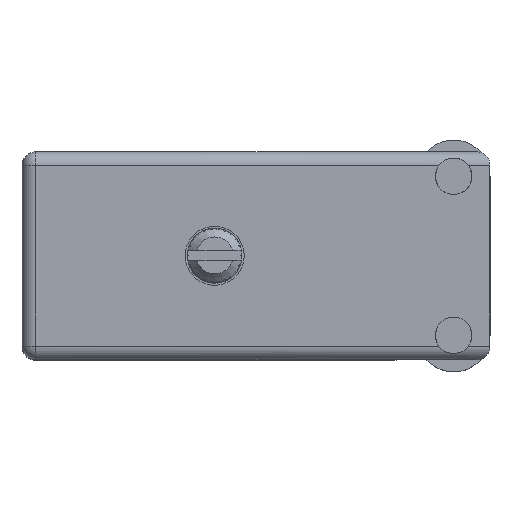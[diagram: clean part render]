
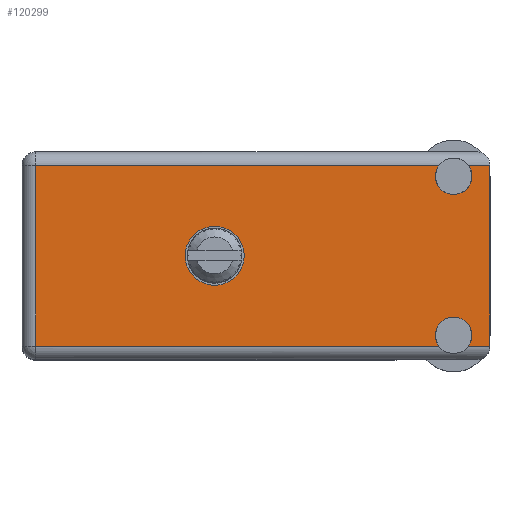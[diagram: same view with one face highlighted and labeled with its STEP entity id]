
A CAD part, top view. The second image highlights one B-rep face of the part: STEP entity #120299.
In plain terms, the highlighted face is planar.
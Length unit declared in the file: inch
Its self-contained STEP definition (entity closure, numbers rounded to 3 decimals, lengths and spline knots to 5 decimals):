
#90 = EDGE_CURVE ( 'NONE', #178435, #7572, #18110, .T. ) ;
#620 = AXIS2_PLACEMENT_3D ( 'NONE', #87096, #186670, #1561 ) ;
#1392 = DIRECTION ( 'NONE',  ( -1., 0., 0. ) ) ;
#1561 = DIRECTION ( 'NONE',  ( 0., 0., 1. ) ) ;
#3412 = FACE_OUTER_BOUND ( 'NONE', #26400, .T. ) ;
#4773 = LINE ( 'NONE', #108244, #90241 ) ;
#5394 = DIRECTION ( 'NONE',  ( 0., 0., 1. ) ) ;
#7572 = VERTEX_POINT ( 'NONE', #61133 ) ;
#8614 = CARTESIAN_POINT ( 'NONE',  ( 0.047, 0.906, -0.668 ) ) ;
#11567 = EDGE_CURVE ( 'NONE', #169026, #52954, #19464, .T. ) ;
#12665 = CARTESIAN_POINT ( 'NONE',  ( 1.609, 0.906, -0.668 ) ) ;
#14396 = VERTEX_POINT ( 'NONE', #134176 ) ;
#15865 = DIRECTION ( 'NONE',  ( 0., 0., 1. ) ) ;
#18110 = LINE ( 'NONE', #146766, #166733 ) ;
#18716 = ORIENTED_EDGE ( 'NONE', *, *, #126770, .F. ) ;
#19232 = CARTESIAN_POINT ( 'NONE',  ( 0.047, 0.906, -0.715 ) ) ;
#19464 = LINE ( 'NONE', #115855, #138938 ) ;
#19802 = CARTESIAN_POINT ( 'NONE',  ( 0.047, 0.906, -0.047 ) ) ;
#20784 = CARTESIAN_POINT ( 'NONE',  ( 0.6625, 0.906, -0.3575 ) ) ;
#24132 = VERTEX_POINT ( 'NONE', #49599 ) ;
#24879 = EDGE_CURVE ( 'NONE', #169026, #179989, #95644, .T. ) ;
#25319 = ORIENTED_EDGE ( 'NONE', *, *, #183548, .T. ) ;
#26400 = EDGE_LOOP ( 'NONE', ( #163845, #70627, #18716, #25319, #99517, #118230, #136854, #134449, #92781, #168842 ) ) ;
#27585 = DIRECTION ( 'NONE',  ( 0., 1., 0. ) ) ;
#30306 = CARTESIAN_POINT ( 'NONE',  ( 1.484, 0.906, -0.631 ) ) ;
#31467 = DIRECTION ( 'NONE',  ( 0., 0., 1. ) ) ;
#36106 = DIRECTION ( 'NONE',  ( 0., 0., 1. ) ) ;
#36639 = DIRECTION ( 'NONE',  ( 1., 0., 0. ) ) ;
#36989 = VECTOR ( 'NONE', #36639, 39.37008 ) ;
#39320 = LINE ( 'NONE', #150470, #36989 ) ;
#39369 = CARTESIAN_POINT ( 'NONE',  ( 0.6625, 0.906, -0.256 ) ) ;
#44323 = CIRCLE ( 'NONE', #620, 0.1015 ) ;
#47089 = ORIENTED_EDGE ( 'NONE', *, *, #61218, .F. ) ;
#48725 = CARTESIAN_POINT ( 'NONE',  ( 1.484, 0.906, -0.084 ) ) ;
#49599 = CARTESIAN_POINT ( 'NONE',  ( 1.43363, 0.906, -0.668 ) ) ;
#52759 = EDGE_CURVE ( 'NONE', #142953, #179690, #44323, .T. ) ;
#52954 = VERTEX_POINT ( 'NONE', #86957 ) ;
#54761 = DIRECTION ( 'NONE',  ( -1., 0., 0. ) ) ;
#55183 = DIRECTION ( 'NONE',  ( 0., 0., 1. ) ) ;
#57534 = VECTOR ( 'NONE', #1392, 39.37008 ) ;
#61133 = CARTESIAN_POINT ( 'NONE',  ( 1.43363, 0.906, -0.047 ) ) ;
#61218 = EDGE_CURVE ( 'NONE', #179690, #142953, #103484, .T. ) ;
#63810 = CARTESIAN_POINT ( 'NONE',  ( 1.53437, 0.906, -0.668 ) ) ;
#69280 = CIRCLE ( 'NONE', #184212, 0.0625 ) ;
#69615 = VECTOR ( 'NONE', #5394, 39.37008 ) ;
#70627 = ORIENTED_EDGE ( 'NONE', *, *, #115244, .F. ) ;
#73059 = AXIS2_PLACEMENT_3D ( 'NONE', #85250, #141267, #55183 ) ;
#77898 = EDGE_CURVE ( 'NONE', #110875, #178435, #107868, .T. ) ;
#82632 = AXIS2_PLACEMENT_3D ( 'NONE', #20784, #120786, #150272 ) ;
#85250 = CARTESIAN_POINT ( 'NONE',  ( 1.484, 0.906, -0.631 ) ) ;
#86957 = CARTESIAN_POINT ( 'NONE',  ( 1.609, 0.906, -0.047 ) ) ;
#87096 = CARTESIAN_POINT ( 'NONE',  ( 0.6625, 0.906, -0.3575 ) ) ;
#87208 = EDGE_CURVE ( 'NONE', #24132, #117075, #146829, .T. ) ;
#90241 = VECTOR ( 'NONE', #54761, 39.37008 ) ;
#92781 = ORIENTED_EDGE ( 'NONE', *, *, #129694, .T. ) ;
#95644 = LINE ( 'NONE', #117705, #57534 ) ;
#99517 = ORIENTED_EDGE ( 'NONE', *, *, #11567, .F. ) ;
#102004 = DIRECTION ( 'NONE',  ( 0., 0., 1. ) ) ;
#103484 = CIRCLE ( 'NONE', #82632, 0.1015 ) ;
#103827 = DIRECTION ( 'NONE',  ( 0., 1., 0. ) ) ;
#105420 = VERTEX_POINT ( 'NONE', #155759 ) ;
#107868 = LINE ( 'NONE', #19232, #69615 ) ;
#108244 = CARTESIAN_POINT ( 'NONE',  ( 0., 0.906, -0.668 ) ) ;
#110875 = VERTEX_POINT ( 'NONE', #8614 ) ;
#114129 = AXIS2_PLACEMENT_3D ( 'NONE', #30306, #130334, #15865 ) ;
#114368 = EDGE_CURVE ( 'NONE', #117075, #179989, #114400, .T. ) ;
#114400 = CIRCLE ( 'NONE', #114129, 0.0625 ) ;
#115244 = EDGE_CURVE ( 'NONE', #105420, #7572, #69280, .T. ) ;
#115615 = CARTESIAN_POINT ( 'NONE',  ( 0., 0.906, -0.715 ) ) ;
#115855 = CARTESIAN_POINT ( 'NONE',  ( 1.609, 0.906, 0. ) ) ;
#117075 = VERTEX_POINT ( 'NONE', #178311 ) ;
#117233 = DIRECTION ( 'NONE',  ( 1., 0., 0. ) ) ;
#117705 = CARTESIAN_POINT ( 'NONE',  ( 0., 0.906, -0.668 ) ) ;
#118230 = ORIENTED_EDGE ( 'NONE', *, *, #24879, .T. ) ;
#120299 = ADVANCED_FACE ( 'NONE', ( #142889, #3412 ), #185593, .T. ) ;
#120786 = DIRECTION ( 'NONE',  ( 0., 1., 0. ) ) ;
#122325 = DIRECTION ( 'NONE',  ( 0., 1., 0. ) ) ;
#126770 = EDGE_CURVE ( 'NONE', #14396, #105420, #167472, .T. ) ;
#126866 = AXIS2_PLACEMENT_3D ( 'NONE', #48725, #122325, #36106 ) ;
#128871 = DIRECTION ( 'NONE',  ( 0., 0., 1. ) ) ;
#129694 = EDGE_CURVE ( 'NONE', #24132, #110875, #4773, .T. ) ;
#130334 = DIRECTION ( 'NONE',  ( 0., 1., 0. ) ) ;
#134176 = CARTESIAN_POINT ( 'NONE',  ( 1.53437, 0.906, -0.047 ) ) ;
#134449 = ORIENTED_EDGE ( 'NONE', *, *, #87208, .F. ) ;
#136854 = ORIENTED_EDGE ( 'NONE', *, *, #114368, .F. ) ;
#138938 = VECTOR ( 'NONE', #102004, 39.37008 ) ;
#141267 = DIRECTION ( 'NONE',  ( 0., 1., 0. ) ) ;
#142889 = FACE_BOUND ( 'NONE', #160147, .T. ) ;
#142953 = VERTEX_POINT ( 'NONE', #167435 ) ;
#144886 = AXIS2_PLACEMENT_3D ( 'NONE', #115615, #27585, #128871 ) ;
#146766 = CARTESIAN_POINT ( 'NONE',  ( 1.609, 0.906, -0.047 ) ) ;
#146829 = CIRCLE ( 'NONE', #73059, 0.0625 ) ;
#150272 = DIRECTION ( 'NONE',  ( 0., 0., 1. ) ) ;
#150470 = CARTESIAN_POINT ( 'NONE',  ( 1.609, 0.906, -0.047 ) ) ;
#155759 = CARTESIAN_POINT ( 'NONE',  ( 1.484, 0.906, -0.1465 ) ) ;
#160147 = EDGE_LOOP ( 'NONE', ( #47089, #162199 ) ) ;
#162199 = ORIENTED_EDGE ( 'NONE', *, *, #52759, .F. ) ;
#163845 = ORIENTED_EDGE ( 'NONE', *, *, #90, .T. ) ;
#166733 = VECTOR ( 'NONE', #117233, 39.37008 ) ;
#167435 = CARTESIAN_POINT ( 'NONE',  ( 0.6625, 0.906, -0.459 ) ) ;
#167472 = CIRCLE ( 'NONE', #126866, 0.0625 ) ;
#168842 = ORIENTED_EDGE ( 'NONE', *, *, #77898, .T. ) ;
#169026 = VERTEX_POINT ( 'NONE', #12665 ) ;
#176238 = CARTESIAN_POINT ( 'NONE',  ( 1.484, 0.906, -0.084 ) ) ;
#178311 = CARTESIAN_POINT ( 'NONE',  ( 1.484, 0.906, -0.5685 ) ) ;
#178435 = VERTEX_POINT ( 'NONE', #19802 ) ;
#179690 = VERTEX_POINT ( 'NONE', #39369 ) ;
#179989 = VERTEX_POINT ( 'NONE', #63810 ) ;
#183548 = EDGE_CURVE ( 'NONE', #14396, #52954, #39320, .T. ) ;
#184212 = AXIS2_PLACEMENT_3D ( 'NONE', #176238, #103827, #31467 ) ;
#185593 = PLANE ( 'NONE',  #144886 ) ;
#186670 = DIRECTION ( 'NONE',  ( 0., 1., 0. ) ) ;
